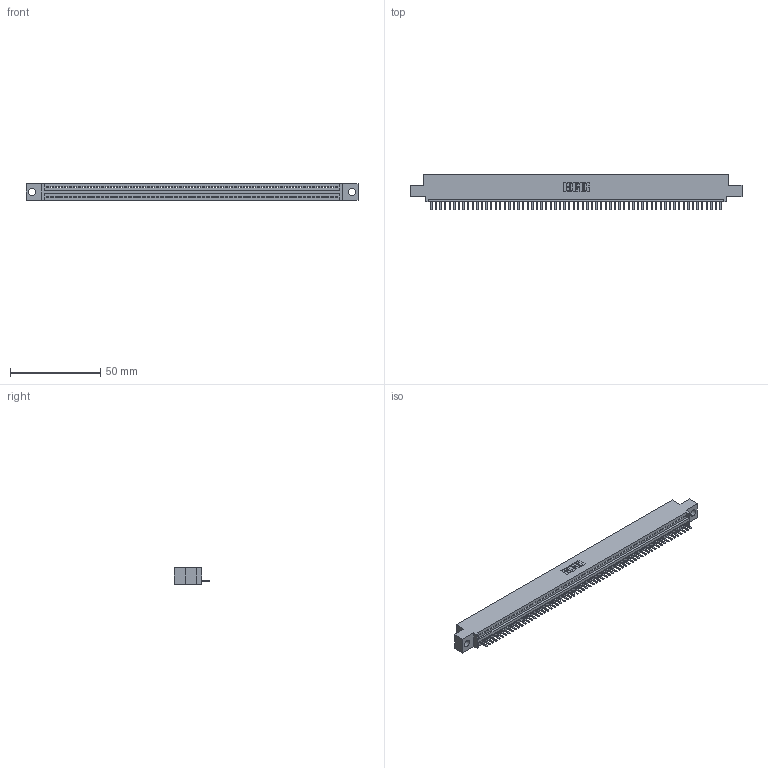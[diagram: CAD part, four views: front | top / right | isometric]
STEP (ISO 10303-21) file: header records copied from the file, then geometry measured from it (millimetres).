
FILE_DESCRIPTION (( 'STEP AP203' ), '1' );
FILE_NAME ('395-064-520-404.STEP', '2019-10-25T00:11:00', ( '' ), ( '' ), 'SwSTEP 2.0', 'SolidWorks 2016', '' );
FILE_SCHEMA (( 'CONFIG_CONTROL_DESIGN' ));
Length unit declared in the file: inch
Products named in the file (3): 395-064-520-404; 345 Part_0.110 Offset - 0.156 Dia-TH; 345-292-001_345-293-120
Assembly tree (65 placements, depth 2):
  395-064-520-404
    345 Part_0.110 Offset - 0.156 Dia-TH
    345-292-001_345-293-120  x64
Bounding box: 183.77 x 19.68 x 9.4 mm (x, y, z)
Volume: 17289.5 mm3; surface area: 22563.5 mm2
Topology: 65 solids, 65 shells, 4098 faces, 12129 edges, 7914 vertices
Faces by surface type: plane 2772, cylinder 1326
Entity records: 45455 total; most frequent: CARTESIAN_POINT 7892, ORIENTED_EDGE 7878, DIRECTION 6847, EDGE_CURVE 3939, LINE 3547, VECTOR 3547, VERTEX_POINT 2622, AXIS2_PLACEMENT_3D 1650
